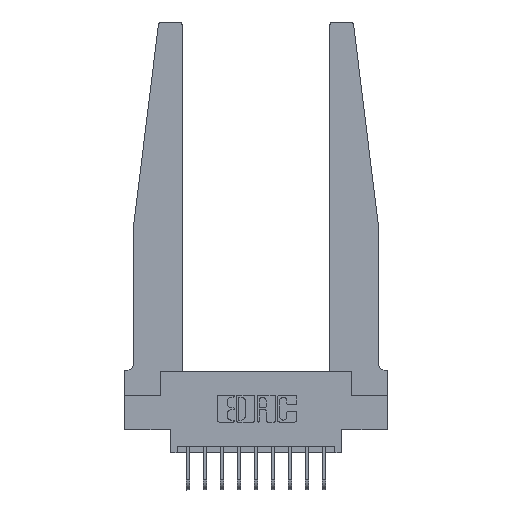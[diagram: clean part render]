
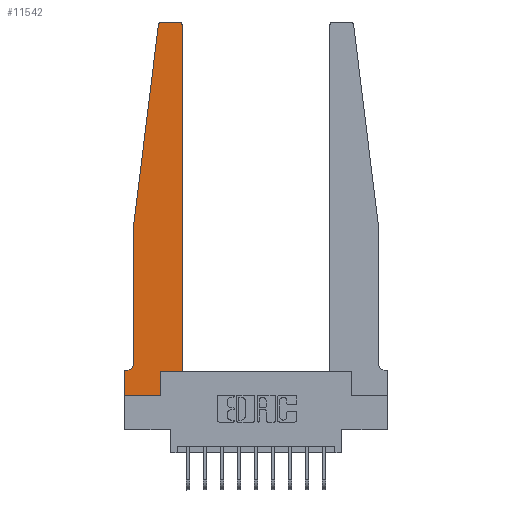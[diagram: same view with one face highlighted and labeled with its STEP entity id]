
A CAD part, top view. The second image highlights one B-rep face of the part: STEP entity #11542.
In plain terms, the highlighted planar face has unit normal (0, 0, 1).
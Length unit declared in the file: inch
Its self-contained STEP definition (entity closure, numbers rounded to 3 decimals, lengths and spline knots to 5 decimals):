
#175 = VECTOR ( 'NONE', #1647, 39.37008 ) ;
#363 = EDGE_CURVE ( 'NONE', #2484, #1329, #3522, .T. ) ;
#500 = ORIENTED_EDGE ( 'NONE', *, *, #10757, .T. ) ;
#586 = CARTESIAN_POINT ( 'NONE',  ( 0.015, 0.2375, 0.37 ) ) ;
#587 = ORIENTED_EDGE ( 'NONE', *, *, #363, .T. ) ;
#663 = DIRECTION ( 'NONE',  ( -1., 0., 0. ) ) ;
#806 = DIRECTION ( 'NONE',  ( 0., -1., 0. ) ) ;
#930 = CARTESIAN_POINT ( 'NONE',  ( 0.27653, 2.72, 0.37 ) ) ;
#964 = CARTESIAN_POINT ( 'NONE',  ( 0.395, 2.75, 0.37 ) ) ;
#1000 = ORIENTED_EDGE ( 'NONE', *, *, #7229, .T. ) ;
#1024 = ORIENTED_EDGE ( 'NONE', *, *, #2609, .T. ) ;
#1182 = CARTESIAN_POINT ( 'NONE',  ( 0., 0., 0.37 ) ) ;
#1213 = VERTEX_POINT ( 'NONE', #13325 ) ;
#1329 = VERTEX_POINT ( 'NONE', #964 ) ;
#1335 = LINE ( 'NONE', #6098, #6557 ) ;
#1397 = CARTESIAN_POINT ( 'NONE',  ( 0.065, 1.25, 0.37 ) ) ;
#1426 = CARTESIAN_POINT ( 'NONE',  ( 0.24675, 2.72367, 0.37 ) ) ;
#1445 = DIRECTION ( 'NONE',  ( -1., 0., 0. ) ) ;
#1448 = VERTEX_POINT ( 'NONE', #1426 ) ;
#1647 = DIRECTION ( 'NONE',  ( 0., 1., 0. ) ) ;
#1676 = VERTEX_POINT ( 'NONE', #8936 ) ;
#1837 = DIRECTION ( 'NONE',  ( 1., 0., 0. ) ) ;
#1970 = LINE ( 'NONE', #11416, #4799 ) ;
#2248 = VECTOR ( 'NONE', #806, 39.37008 ) ;
#2268 = DIRECTION ( 'NONE',  ( 1., 0., 0. ) ) ;
#2484 = VERTEX_POINT ( 'NONE', #15352 ) ;
#2609 = EDGE_CURVE ( 'NONE', #9812, #11119, #15024, .T. ) ;
#2670 = VERTEX_POINT ( 'NONE', #4723 ) ;
#3134 = VECTOR ( 'NONE', #2268, 39.37008 ) ;
#3185 = DIRECTION ( 'NONE',  ( 0., 0., 1. ) ) ;
#3382 = PLANE ( 'NONE',  #10801 ) ;
#3405 = CARTESIAN_POINT ( 'NONE',  ( 0.425, 0.18, 0.37 ) ) ;
#3451 = ORIENTED_EDGE ( 'NONE', *, *, #11404, .T. ) ;
#3522 = CIRCLE ( 'NONE', #5513, 0.03 ) ;
#3890 = VERTEX_POINT ( 'NONE', #10412 ) ;
#3974 = CARTESIAN_POINT ( 'NONE',  ( 0.065, 0.1875, 0.37 ) ) ;
#4122 = VECTOR ( 'NONE', #15078, 39.37008 ) ;
#4685 = EDGE_CURVE ( 'NONE', #10914, #13525, #12262, .T. ) ;
#4723 = CARTESIAN_POINT ( 'NONE',  ( 0.065, 0.2375, 0.37 ) ) ;
#4799 = VECTOR ( 'NONE', #5587, 39.37008 ) ;
#5217 = DIRECTION ( 'NONE',  ( 0., 0., -1. ) ) ;
#5219 = CARTESIAN_POINT ( 'NONE',  ( 0., 0.1875, 0.37 ) ) ;
#5440 = DIRECTION ( 'NONE',  ( 0., 0., 1. ) ) ;
#5513 = AXIS2_PLACEMENT_3D ( 'NONE', #11648, #3185, #6809 ) ;
#5548 = VECTOR ( 'NONE', #15153, 39.37008 ) ;
#5571 = AXIS2_PLACEMENT_3D ( 'NONE', #930, #10438, #13843 ) ;
#5587 = DIRECTION ( 'NONE',  ( 0., 1., 0. ) ) ;
#5682 = EDGE_CURVE ( 'NONE', #3890, #9812, #13237, .T. ) ;
#5719 = EDGE_CURVE ( 'NONE', #8874, #2670, #7536, .T. ) ;
#5861 = LINE ( 'NONE', #8167, #5548 ) ;
#6098 = CARTESIAN_POINT ( 'NONE',  ( 0.065, 1.25, 0.37 ) ) ;
#6557 = VECTOR ( 'NONE', #10843, 39.37008 ) ;
#6628 = CARTESIAN_POINT ( 'NONE',  ( 0., 0., 0.37 ) ) ;
#6648 = ORIENTED_EDGE ( 'NONE', *, *, #14510, .T. ) ;
#6809 = DIRECTION ( 'NONE',  ( 1., 0., 0. ) ) ;
#7229 = EDGE_CURVE ( 'NONE', #1213, #2484, #1970, .T. ) ;
#7351 = CARTESIAN_POINT ( 'NONE',  ( 0., 0.1875, 0.37 ) ) ;
#7405 = VECTOR ( 'NONE', #1445, 39.37008 ) ;
#7448 = CARTESIAN_POINT ( 'NONE',  ( 0.065, 1.25, 0.37 ) ) ;
#7535 = CIRCLE ( 'NONE', #5571, 0.03 ) ;
#7536 = LINE ( 'NONE', #7448, #15154 ) ;
#7697 = DIRECTION ( 'NONE',  ( 0., -1., 0. ) ) ;
#7796 = CARTESIAN_POINT ( 'NONE',  ( 0.2605, 0.18, 0.37 ) ) ;
#7974 = CARTESIAN_POINT ( 'NONE',  ( 0., 0., 0.37 ) ) ;
#8112 = ORIENTED_EDGE ( 'NONE', *, *, #14842, .T. ) ;
#8167 = CARTESIAN_POINT ( 'NONE',  ( 0.25, 2.75, 0.37 ) ) ;
#8750 = CARTESIAN_POINT ( 'NONE',  ( 0.2605, 0.18, 0.37 ) ) ;
#8874 = VERTEX_POINT ( 'NONE', #1397 ) ;
#8936 = CARTESIAN_POINT ( 'NONE',  ( 0.27653, 2.75, 0.37 ) ) ;
#9202 = ORIENTED_EDGE ( 'NONE', *, *, #4685, .T. ) ;
#9812 = VERTEX_POINT ( 'NONE', #7351 ) ;
#10096 = ORIENTED_EDGE ( 'NONE', *, *, #13364, .T. ) ;
#10412 = CARTESIAN_POINT ( 'NONE',  ( 0.015, 0.1875, 0.37 ) ) ;
#10438 = DIRECTION ( 'NONE',  ( 0., 0., 1. ) ) ;
#10757 = EDGE_CURVE ( 'NONE', #2670, #3890, #14040, .T. ) ;
#10782 = CARTESIAN_POINT ( 'NONE',  ( 0.2605, 0., 0.37 ) ) ;
#10801 = AXIS2_PLACEMENT_3D ( 'NONE', #5219, #5440, #1837 ) ;
#10843 = DIRECTION ( 'NONE',  ( -0.122, -0.992, 0. ) ) ;
#10914 = VERTEX_POINT ( 'NONE', #10782 ) ;
#11017 = ORIENTED_EDGE ( 'NONE', *, *, #5719, .T. ) ;
#11119 = VERTEX_POINT ( 'NONE', #1182 ) ;
#11133 = ORIENTED_EDGE ( 'NONE', *, *, #12581, .T. ) ;
#11404 = EDGE_CURVE ( 'NONE', #11119, #10914, #15148, .T. ) ;
#11416 = CARTESIAN_POINT ( 'NONE',  ( 0.425, 0.18, 0.37 ) ) ;
#11542 = ADVANCED_FACE ( 'NONE', ( #14048 ), #3382, .T. ) ;
#11648 = CARTESIAN_POINT ( 'NONE',  ( 0.395, 2.72, 0.37 ) ) ;
#12262 = LINE ( 'NONE', #8750, #175 ) ;
#12518 = EDGE_LOOP ( 'NONE', ( #8112, #11133, #10096, #11017, #500, #14133, #1024, #3451, #9202, #6648, #1000, #587 ) ) ;
#12581 = EDGE_CURVE ( 'NONE', #1676, #1448, #7535, .T. ) ;
#13237 = LINE ( 'NONE', #3974, #7405 ) ;
#13325 = CARTESIAN_POINT ( 'NONE',  ( 0.425, 0.18, 0.37 ) ) ;
#13364 = EDGE_CURVE ( 'NONE', #1448, #8874, #1335, .T. ) ;
#13525 = VERTEX_POINT ( 'NONE', #7796 ) ;
#13554 = AXIS2_PLACEMENT_3D ( 'NONE', #586, #5217, #663 ) ;
#13843 = DIRECTION ( 'NONE',  ( 1., 0., 0. ) ) ;
#14040 = CIRCLE ( 'NONE', #13554, 0.05 ) ;
#14048 = FACE_OUTER_BOUND ( 'NONE', #12518, .T. ) ;
#14073 = LINE ( 'NONE', #3405, #3134 ) ;
#14133 = ORIENTED_EDGE ( 'NONE', *, *, #5682, .T. ) ;
#14510 = EDGE_CURVE ( 'NONE', #13525, #1213, #14073, .T. ) ;
#14842 = EDGE_CURVE ( 'NONE', #1329, #1676, #5861, .T. ) ;
#15024 = LINE ( 'NONE', #7974, #2248 ) ;
#15078 = DIRECTION ( 'NONE',  ( 1., 0., 0. ) ) ;
#15148 = LINE ( 'NONE', #6628, #4122 ) ;
#15153 = DIRECTION ( 'NONE',  ( -1., 0., 0. ) ) ;
#15154 = VECTOR ( 'NONE', #7697, 39.37008 ) ;
#15352 = CARTESIAN_POINT ( 'NONE',  ( 0.425, 2.72, 0.37 ) ) ;
